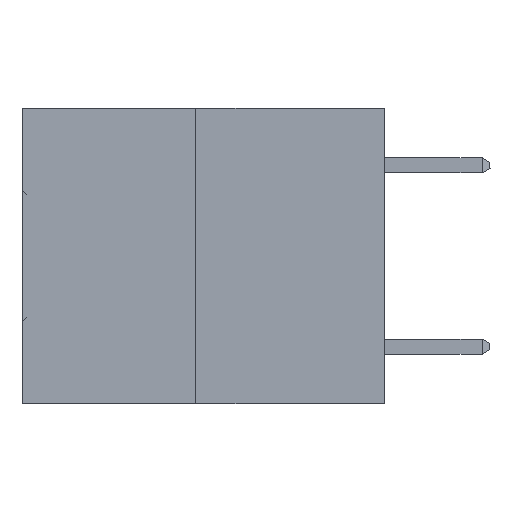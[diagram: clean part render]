
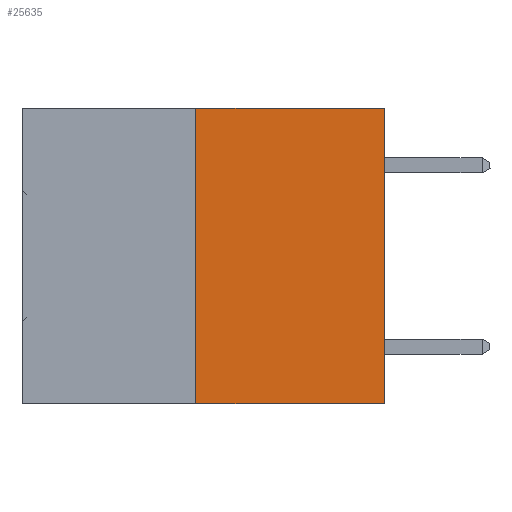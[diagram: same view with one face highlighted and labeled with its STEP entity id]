
A CAD part, left-side view. The second image highlights one B-rep face of the part: STEP entity #25635.
In plain terms, the highlighted planar face has unit normal (-1, 0, 0).
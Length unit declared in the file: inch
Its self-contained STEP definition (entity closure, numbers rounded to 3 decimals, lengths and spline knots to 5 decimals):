
#242 = CARTESIAN_POINT ( 'NONE',  ( 0., 0.6, 0. ) ) ;
#361 = VERTEX_POINT ( 'NONE', #21535 ) ;
#378 = DIRECTION ( 'NONE',  ( 0., -1., 0. ) ) ;
#2041 = CARTESIAN_POINT ( 'NONE',  ( 0., 0.6, -0.49 ) ) ;
#2267 = VECTOR ( 'NONE', #378, 39.37008 ) ;
#3300 = FACE_OUTER_BOUND ( 'NONE', #11793, .T. ) ;
#4376 = EDGE_CURVE ( 'NONE', #361, #13857, #15369, .T. ) ;
#4399 = DIRECTION ( 'NONE',  ( 0., 0., 1. ) ) ;
#4402 = CARTESIAN_POINT ( 'NONE',  ( 0., 0.6, 0. ) ) ;
#5131 = LINE ( 'NONE', #2041, #14309 ) ;
#7957 = DIRECTION ( 'NONE',  ( 0., 0., 1. ) ) ;
#10448 = DIRECTION ( 'NONE',  ( 1., 0., 0. ) ) ;
#11058 = CARTESIAN_POINT ( 'NONE',  ( 0., 0., 0. ) ) ;
#11793 = EDGE_LOOP ( 'NONE', ( #12808, #34538, #25124, #25353 ) ) ;
#12808 = ORIENTED_EDGE ( 'NONE', *, *, #4376, .F. ) ;
#13857 = VERTEX_POINT ( 'NONE', #18378 ) ;
#14309 = VECTOR ( 'NONE', #28435, 39.37008 ) ;
#14345 = VECTOR ( 'NONE', #7957, 39.37008 ) ;
#15369 = LINE ( 'NONE', #15475, #27671 ) ;
#15475 = CARTESIAN_POINT ( 'NONE',  ( 0., 0.312, -0.49 ) ) ;
#15882 = VERTEX_POINT ( 'NONE', #17386 ) ;
#16349 = DIRECTION ( 'NONE',  ( 0., 0., -1. ) ) ;
#17212 = VERTEX_POINT ( 'NONE', #24588 ) ;
#17386 = CARTESIAN_POINT ( 'NONE',  ( 0., 0., -0.49 ) ) ;
#18378 = CARTESIAN_POINT ( 'NONE',  ( 0., 0.312, 0. ) ) ;
#19205 = AXIS2_PLACEMENT_3D ( 'NONE', #4402, #10448, #16349 ) ;
#21535 = CARTESIAN_POINT ( 'NONE',  ( 0., 0.312, -0.49 ) ) ;
#22085 = LINE ( 'NONE', #11058, #14345 ) ;
#24588 = CARTESIAN_POINT ( 'NONE',  ( 0., 0., 0. ) ) ;
#25124 = ORIENTED_EDGE ( 'NONE', *, *, #34068, .T. ) ;
#25176 = EDGE_CURVE ( 'NONE', #361, #15882, #5131, .T. ) ;
#25353 = ORIENTED_EDGE ( 'NONE', *, *, #26792, .F. ) ;
#25635 = ADVANCED_FACE ( 'NONE', ( #3300 ), #28193, .F. ) ;
#26792 = EDGE_CURVE ( 'NONE', #13857, #17212, #35767, .T. ) ;
#27671 = VECTOR ( 'NONE', #4399, 39.37008 ) ;
#28193 = PLANE ( 'NONE',  #19205 ) ;
#28435 = DIRECTION ( 'NONE',  ( 0., -1., 0. ) ) ;
#34068 = EDGE_CURVE ( 'NONE', #15882, #17212, #22085, .T. ) ;
#34538 = ORIENTED_EDGE ( 'NONE', *, *, #25176, .T. ) ;
#35767 = LINE ( 'NONE', #242, #2267 ) ;
